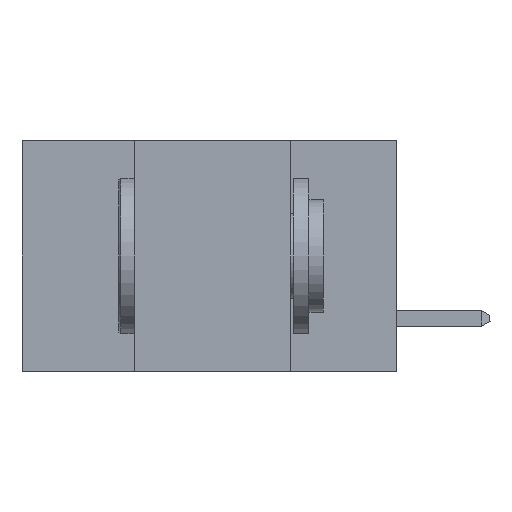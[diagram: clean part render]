
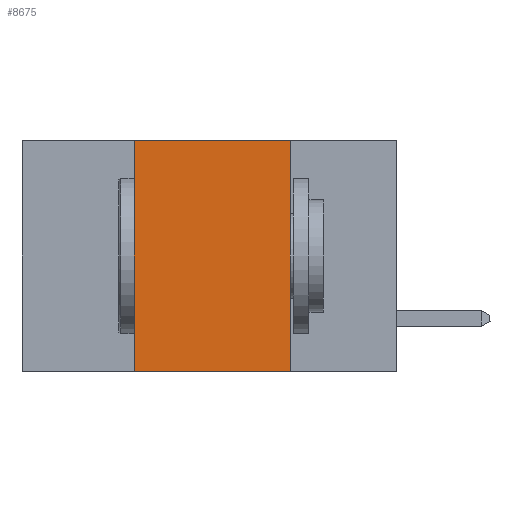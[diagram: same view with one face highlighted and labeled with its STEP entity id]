
A CAD part, left-side view. The second image highlights one B-rep face of the part: STEP entity #8675.
In plain terms, the highlighted planar face has unit normal (-1, 0, 0).
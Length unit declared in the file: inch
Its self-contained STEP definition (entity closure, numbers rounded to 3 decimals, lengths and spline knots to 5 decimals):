
#564 = ORIENTED_EDGE ( 'NONE', *, *, #11475, .F. ) ;
#734 = VECTOR ( 'NONE', #14892, 39.37008 ) ;
#856 = EDGE_CURVE ( 'NONE', #16305, #19252, #17944, .T. ) ;
#1169 = ORIENTED_EDGE ( 'NONE', *, *, #14383, .F. ) ;
#1188 = CARTESIAN_POINT ( 'NONE',  ( 0., 0.42, 0. ) ) ;
#1546 = VECTOR ( 'NONE', #17633, 39.37008 ) ;
#1858 = ORIENTED_EDGE ( 'NONE', *, *, #856, .F. ) ;
#2755 = VERTEX_POINT ( 'NONE', #18739 ) ;
#2937 = LINE ( 'NONE', #5343, #10908 ) ;
#3837 = CARTESIAN_POINT ( 'NONE',  ( 0., 0.6, -0.37 ) ) ;
#4401 = PLANE ( 'NONE',  #10646 ) ;
#4484 = VERTEX_POINT ( 'NONE', #10691 ) ;
#4569 = DIRECTION ( 'NONE',  ( 0., 0., 1. ) ) ;
#5343 = CARTESIAN_POINT ( 'NONE',  ( 0., 0.6, 0. ) ) ;
#5390 = CARTESIAN_POINT ( 'NONE',  ( 0., 0.42, -0.37 ) ) ;
#6029 = DIRECTION ( 'NONE',  ( 0., 0., -1. ) ) ;
#8675 = ADVANCED_FACE ( 'NONE', ( #16573 ), #4401, .F. ) ;
#10010 = LINE ( 'NONE', #19185, #1546 ) ;
#10646 = AXIS2_PLACEMENT_3D ( 'NONE', #18546, #15456, #6029 ) ;
#10691 = CARTESIAN_POINT ( 'NONE',  ( 0., 0.17, -0.37 ) ) ;
#10908 = VECTOR ( 'NONE', #19476, 39.37008 ) ;
#11475 = EDGE_CURVE ( 'NONE', #19252, #2755, #2937, .T. ) ;
#12857 = CARTESIAN_POINT ( 'NONE',  ( 0., 0.42, 0. ) ) ;
#13352 = ORIENTED_EDGE ( 'NONE', *, *, #19457, .T. ) ;
#14383 = EDGE_CURVE ( 'NONE', #2755, #4484, #10010, .T. ) ;
#14892 = DIRECTION ( 'NONE',  ( 0., -1., 0. ) ) ;
#15456 = DIRECTION ( 'NONE',  ( 1., 0., 0. ) ) ;
#16305 = VERTEX_POINT ( 'NONE', #5390 ) ;
#16573 = FACE_OUTER_BOUND ( 'NONE', #19401, .T. ) ;
#17040 = LINE ( 'NONE', #3837, #734 ) ;
#17633 = DIRECTION ( 'NONE',  ( 0., 0., -1. ) ) ;
#17944 = LINE ( 'NONE', #1188, #18436 ) ;
#18436 = VECTOR ( 'NONE', #4569, 39.37008 ) ;
#18546 = CARTESIAN_POINT ( 'NONE',  ( 0., 0.6, 0. ) ) ;
#18739 = CARTESIAN_POINT ( 'NONE',  ( 0., 0.17, 0. ) ) ;
#19185 = CARTESIAN_POINT ( 'NONE',  ( 0., 0.17, 0. ) ) ;
#19252 = VERTEX_POINT ( 'NONE', #12857 ) ;
#19401 = EDGE_LOOP ( 'NONE', ( #1169, #564, #1858, #13352 ) ) ;
#19457 = EDGE_CURVE ( 'NONE', #16305, #4484, #17040, .T. ) ;
#19476 = DIRECTION ( 'NONE',  ( 0., -1., 0. ) ) ;
